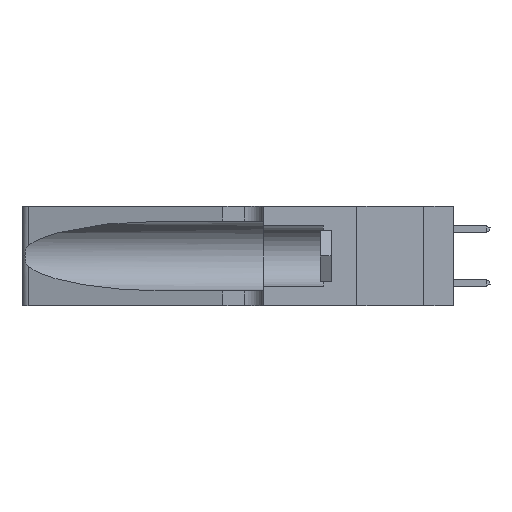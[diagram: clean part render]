
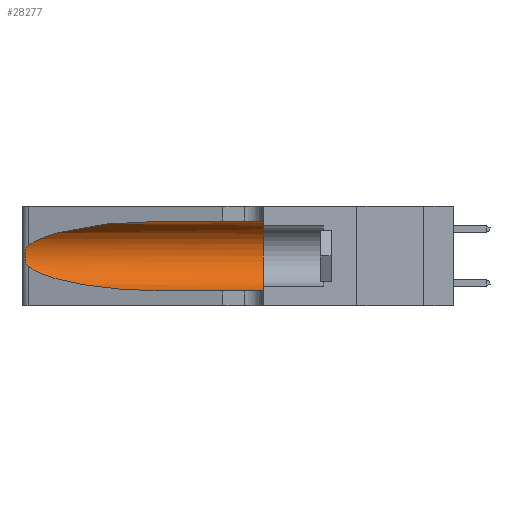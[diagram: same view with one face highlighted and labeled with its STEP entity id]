
A CAD part, left-side view. The second image highlights one B-rep face of the part: STEP entity #28277.
In plain terms, the highlighted cylindrical face has radius 3.308 mm (diameter 6.617 mm), a partial arc.
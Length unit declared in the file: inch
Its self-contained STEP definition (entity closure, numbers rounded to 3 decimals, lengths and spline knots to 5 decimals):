
#565 = B_SPLINE_CURVE_WITH_KNOTS ( 'NONE', 3,
 ( #15717, #36217, #22563, #1952, #26009, #5451, #29460, #8907, #32914, #12376, #36357, #15866, #39766, #19269 ),
 .UNSPECIFIED., .F., .F.,
 ( 4, 2, 2, 2, 2, 2, 4 ),
 ( 0., 0.00027, 0.00053, 0.00107, 0.0016, 0.00187, 0.00214 ),
 .UNSPECIFIED. ) ;
#860 = VERTEX_POINT ( 'NONE', #37074 ) ;
#1952 = CARTESIAN_POINT ( 'NONE',  ( 0.25787, 1.23484, 0.2124 ) ) ;
#2073 = VECTOR ( 'NONE', #16435, 39.37008 ) ;
#3085 = EDGE_CURVE ( 'NONE', #36105, #860, #565, .T. ) ;
#4870 = CARTESIAN_POINT ( 'NONE',  ( 0.25487, 1.22718, 0.22369 ) ) ;
#5451 = CARTESIAN_POINT ( 'NONE',  ( 0.26018, 1.23835, 0.19895 ) ) ;
#5577 = ORIENTED_EDGE ( 'NONE', *, *, #44050, .F. ) ;
#5832 = EDGE_CURVE ( 'NONE', #24497, #7980, #35418, .T. ) ;
#6660 = VERTEX_POINT ( 'NONE', #37464 ) ;
#6727 = CARTESIAN_POINT ( 'NONE',  ( 0.1305, 1.61858, 0.31525 ) ) ;
#7230 = FACE_OUTER_BOUND ( 'NONE', #40139, .T. ) ;
#7237 = CARTESIAN_POINT ( 'NONE',  ( 0.1305, 0.35, 0.05475 ) ) ;
#7510 = ORIENTED_EDGE ( 'NONE', *, *, #40520, .T. ) ;
#7980 = VERTEX_POINT ( 'NONE', #7237 ) ;
#8907 = CARTESIAN_POINT ( 'NONE',  ( 0.26075, 1.23896, 0.178 ) ) ;
#9660 = CARTESIAN_POINT ( 'NONE',  ( 0.1305, 0.35, 0.31525 ) ) ;
#9697 = CARTESIAN_POINT ( 'NONE',  ( 0.25487, 1.22718, 0.22369 ) ) ;
#10191 = DIRECTION ( 'NONE',  ( 0., -1., 0. ) ) ;
#11678 = CARTESIAN_POINT ( 'NONE',  ( 0.1305, 0.35, 0.185 ) ) ;
#12376 = CARTESIAN_POINT ( 'NONE',  ( 0.25856, 1.23593, 0.16098 ) ) ;
#15025 = DIRECTION ( 'NONE',  ( 0., 0., -1. ) ) ;
#15154 = DIRECTION ( 'NONE',  ( 0., 0., 1. ) ) ;
#15332 = CYLINDRICAL_SURFACE ( 'NONE', #21704, 0.13025 ) ;
#15717 = CARTESIAN_POINT ( 'NONE',  ( 0.25487, 1.22718, 0.22369 ) ) ;
#15866 = CARTESIAN_POINT ( 'NONE',  ( 0.25639, 1.23186, 0.15144 ) ) ;
#16435 = DIRECTION ( 'NONE',  ( 0., -1., 0. ) ) ;
#17008 = VECTOR ( 'NONE', #10191, 39.37008 ) ;
#19140 = EDGE_CURVE ( 'NONE', #20043, #7980, #21544, .T. ) ;
#19269 = CARTESIAN_POINT ( 'NONE',  ( 0.25487, 1.22718, 0.14631 ) ) ;
#19852 = CARTESIAN_POINT ( 'NONE',  ( 0.18966, 0.96281, 0.05475 ) ) ;
#20043 = VERTEX_POINT ( 'NONE', #9660 ) ;
#21544 = CIRCLE ( 'NONE', #27207, 0.13025 ) ;
#21704 = AXIS2_PLACEMENT_3D ( 'NONE', #28639, #35528, #15025 ) ;
#22563 = CARTESIAN_POINT ( 'NONE',  ( 0.25639, 1.23184, 0.21858 ) ) ;
#24497 = VERTEX_POINT ( 'NONE', #37445 ) ;
#25942 =( BOUNDED_CURVE ( )  B_SPLINE_CURVE ( 3, ( #33517, #36925, #19852, #43745 ),
 .UNSPECIFIED., .F., .T. ) 
 B_SPLINE_CURVE_WITH_KNOTS ( ( 4, 4 ),
 ( 3.44316, 4.71239 ),
 .UNSPECIFIED. ) 
 CURVE ( )  GEOMETRIC_REPRESENTATION_ITEM ( )  RATIONAL_B_SPLINE_CURVE ( ( 1., 0.87, 0.87, 1. ) ) 
 REPRESENTATION_ITEM ( '' )  );
#26009 = CARTESIAN_POINT ( 'NONE',  ( 0.25854, 1.2359, 0.20912 ) ) ;
#26557 = ORIENTED_EDGE ( 'NONE', *, *, #19140, .F. ) ;
#26782 = CARTESIAN_POINT ( 'NONE',  ( 0.1305, 0.72297, 0.31525 ) ) ;
#27207 = AXIS2_PLACEMENT_3D ( 'NONE', #11678, #35653, #15154 ) ;
#28260 = LINE ( 'NONE', #6727, #17008 ) ;
#28277 = ADVANCED_FACE ( 'NONE', ( #7230 ), #15332, .F. ) ;
#28639 = CARTESIAN_POINT ( 'NONE',  ( 0.1305, 1.61858, 0.185 ) ) ;
#28887 = ORIENTED_EDGE ( 'NONE', *, *, #40039, .T. ) ;
#29460 = CARTESIAN_POINT ( 'NONE',  ( 0.26075, 1.23896, 0.19203 ) ) ;
#30244 = CARTESIAN_POINT ( 'NONE',  ( 0.2373, 1.15595, 0.28018 ) ) ;
#32914 = CARTESIAN_POINT ( 'NONE',  ( 0.26017, 1.23833, 0.17102 ) ) ;
#33517 = CARTESIAN_POINT ( 'NONE',  ( 0.25487, 1.22718, 0.14631 ) ) ;
#35418 = LINE ( 'NONE', #36915, #2073 ) ;
#35528 = DIRECTION ( 'NONE',  ( 0., -1., 0. ) ) ;
#35653 = DIRECTION ( 'NONE',  ( 0., 1., 0. ) ) ;
#36105 = VERTEX_POINT ( 'NONE', #4870 ) ;
#36217 = CARTESIAN_POINT ( 'NONE',  ( 0.25555, 1.22994, 0.2215 ) ) ;
#36357 = CARTESIAN_POINT ( 'NONE',  ( 0.25789, 1.23486, 0.15765 ) ) ;
#36915 = CARTESIAN_POINT ( 'NONE',  ( 0.1305, 1.61858, 0.05475 ) ) ;
#36925 = CARTESIAN_POINT ( 'NONE',  ( 0.2373, 1.15595, 0.08982 ) ) ;
#37074 = CARTESIAN_POINT ( 'NONE',  ( 0.25487, 1.22718, 0.14631 ) ) ;
#37445 = CARTESIAN_POINT ( 'NONE',  ( 0.1305, 0.72297, 0.05475 ) ) ;
#37464 = CARTESIAN_POINT ( 'NONE',  ( 0.1305, 0.72297, 0.31525 ) ) ;
#39766 = CARTESIAN_POINT ( 'NONE',  ( 0.25555, 1.22993, 0.14849 ) ) ;
#40039 = EDGE_CURVE ( 'NONE', #6660, #36105, #41799, .T. ) ;
#40139 = EDGE_LOOP ( 'NONE', ( #28887, #43446, #7510, #41353, #26557, #5577 ) ) ;
#40398 = CARTESIAN_POINT ( 'NONE',  ( 0.18966, 0.96281, 0.31525 ) ) ;
#40520 = EDGE_CURVE ( 'NONE', #860, #24497, #25942, .T. ) ;
#41353 = ORIENTED_EDGE ( 'NONE', *, *, #5832, .T. ) ;
#41799 =( BOUNDED_CURVE ( )  B_SPLINE_CURVE ( 3, ( #26782, #40398, #30244, #9697 ),
 .UNSPECIFIED., .F., .F. ) 
 B_SPLINE_CURVE_WITH_KNOTS ( ( 4, 4 ),
 ( 1.5708, 2.84003 ),
 .UNSPECIFIED. ) 
 CURVE ( )  GEOMETRIC_REPRESENTATION_ITEM ( )  RATIONAL_B_SPLINE_CURVE ( ( 1., 0.87, 0.87, 1. ) ) 
 REPRESENTATION_ITEM ( '' )  );
#43446 = ORIENTED_EDGE ( 'NONE', *, *, #3085, .T. ) ;
#43745 = CARTESIAN_POINT ( 'NONE',  ( 0.1305, 0.72297, 0.05475 ) ) ;
#44050 = EDGE_CURVE ( 'NONE', #6660, #20043, #28260, .T. ) ;
